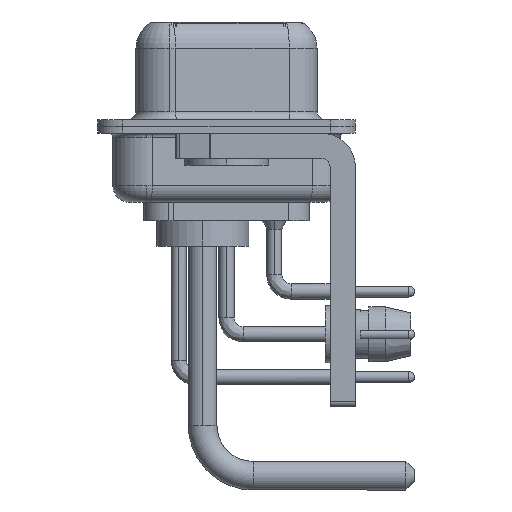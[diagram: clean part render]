
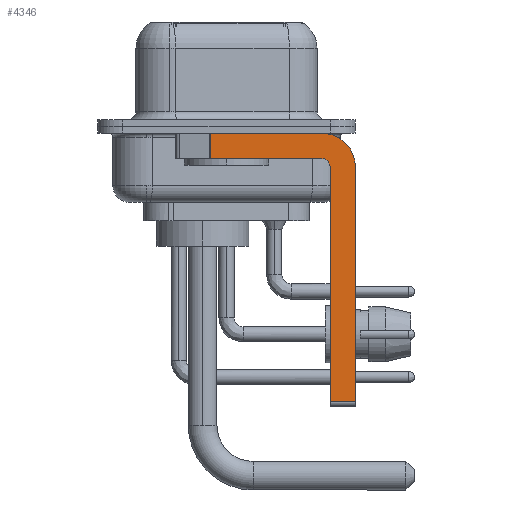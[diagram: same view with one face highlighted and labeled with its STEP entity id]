
A CAD part, left-side view. The second image highlights one B-rep face of the part: STEP entity #4346.
In plain terms, the highlighted planar face has unit normal (-1, 0, 0).
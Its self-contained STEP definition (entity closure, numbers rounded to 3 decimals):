
#274 = EDGE_CURVE ( 'NONE', #16400, #15756, #26025, .T. ) ;
#583 = EDGE_CURVE ( 'NONE', #9301, #2854, #10299, .T. ) ;
#618 = EDGE_CURVE ( 'NONE', #28254, #19054, #13536, .T. ) ;
#1569 = EDGE_CURVE ( 'NONE', #19054, #15756, #11273, .T. ) ;
#2556 = PLANE ( 'NONE',  #16805 ) ;
#2561 = VERTEX_POINT ( 'NONE', #9936 ) ;
#2715 = DIRECTION ( 'NONE',  ( 0., 0., 1. ) ) ;
#2854 = VERTEX_POINT ( 'NONE', #19537 ) ;
#3910 = DIRECTION ( 'NONE',  ( 0., 1., 0. ) ) ;
#4150 = EDGE_CURVE ( 'NONE', #2561, #2854, #21300, .T. ) ;
#4299 = VECTOR ( 'NONE', #22179, 1000. ) ;
#4346 = ADVANCED_FACE ( 'NONE', ( #14711 ), #2556, .F. ) ;
#4815 = ORIENTED_EDGE ( 'NONE', *, *, #618, .F. ) ;
#4873 = DIRECTION ( 'NONE',  ( 1., 0., 0. ) ) ;
#5376 = AXIS2_PLACEMENT_3D ( 'NONE', #22661, #20247, #10449 ) ;
#5695 = VECTOR ( 'NONE', #3910, 1000. ) ;
#6154 = CARTESIAN_POINT ( 'NONE',  ( -2.9, 0.978, -1.9 ) ) ;
#6637 = VECTOR ( 'NONE', #8551, 1000. ) ;
#7139 = VECTOR ( 'NONE', #14784, 1000. ) ;
#8011 = ORIENTED_EDGE ( 'NONE', *, *, #20557, .F. ) ;
#8551 = DIRECTION ( 'NONE',  ( 0., 0., -1. ) ) ;
#8844 = CIRCLE ( 'NONE', #9340, 2. ) ;
#9301 = VERTEX_POINT ( 'NONE', #30287 ) ;
#9340 = AXIS2_PLACEMENT_3D ( 'NONE', #26995, #4873, #14967 ) ;
#9581 = DIRECTION ( 'NONE',  ( 1., 0., 0. ) ) ;
#9936 = CARTESIAN_POINT ( 'NONE',  ( -2.9, -7.65, -2.4 ) ) ;
#9982 = CARTESIAN_POINT ( 'NONE',  ( -2.9, -5.65, -16.35 ) ) ;
#9999 = EDGE_CURVE ( 'NONE', #9301, #28254, #22275, .T. ) ;
#10299 = LINE ( 'NONE', #9982, #4299 ) ;
#10449 = DIRECTION ( 'NONE',  ( 0., 0., 1. ) ) ;
#10616 = VECTOR ( 'NONE', #16011, 1000. ) ;
#10702 = VERTEX_POINT ( 'NONE', #15596 ) ;
#10873 = CARTESIAN_POINT ( 'NONE',  ( -2.9, -7.65, -2.4 ) ) ;
#10955 = CARTESIAN_POINT ( 'NONE',  ( -2.9, -5.65, -1.9 ) ) ;
#11273 = LINE ( 'NONE', #10955, #5695 ) ;
#12089 = CARTESIAN_POINT ( 'NONE',  ( -2.9, -6.15, -2.4 ) ) ;
#12495 = ORIENTED_EDGE ( 'NONE', *, *, #1569, .F. ) ;
#13536 = CIRCLE ( 'NONE', #5376, 0.5 ) ;
#14338 = ORIENTED_EDGE ( 'NONE', *, *, #4150, .F. ) ;
#14711 = FACE_OUTER_BOUND ( 'NONE', #17903, .T. ) ;
#14784 = DIRECTION ( 'NONE',  ( 0., -1., 0. ) ) ;
#14967 = DIRECTION ( 'NONE',  ( 0., 0., -1. ) ) ;
#15596 = CARTESIAN_POINT ( 'NONE',  ( -2.9, -5.65, -0.4 ) ) ;
#15642 = ORIENTED_EDGE ( 'NONE', *, *, #583, .T. ) ;
#15756 = VERTEX_POINT ( 'NONE', #29394 ) ;
#16011 = DIRECTION ( 'NONE',  ( 0., 0., -1. ) ) ;
#16400 = VERTEX_POINT ( 'NONE', #18113 ) ;
#16805 = AXIS2_PLACEMENT_3D ( 'NONE', #31576, #9581, #19217 ) ;
#17903 = EDGE_LOOP ( 'NONE', ( #8011, #23789, #12495, #4815, #29987, #15642, #14338, #29711 ) ) ;
#18113 = CARTESIAN_POINT ( 'NONE',  ( -2.9, 0.978, -0.4 ) ) ;
#19054 = VERTEX_POINT ( 'NONE', #31001 ) ;
#19217 = DIRECTION ( 'NONE',  ( 0., 0., -1. ) ) ;
#19537 = CARTESIAN_POINT ( 'NONE',  ( -2.9, -7.65, -16.35 ) ) ;
#20247 = DIRECTION ( 'NONE',  ( -1., 0., 0. ) ) ;
#20557 = EDGE_CURVE ( 'NONE', #16400, #10702, #24577, .T. ) ;
#21300 = LINE ( 'NONE', #10873, #10616 ) ;
#22179 = DIRECTION ( 'NONE',  ( 0., -1., 0. ) ) ;
#22275 = LINE ( 'NONE', #24514, #26876 ) ;
#22661 = CARTESIAN_POINT ( 'NONE',  ( -2.9, -5.65, -2.4 ) ) ;
#23789 = ORIENTED_EDGE ( 'NONE', *, *, #274, .T. ) ;
#23838 = EDGE_CURVE ( 'NONE', #10702, #2561, #8844, .T. ) ;
#24514 = CARTESIAN_POINT ( 'NONE',  ( -2.9, -6.15, -16.6 ) ) ;
#24577 = LINE ( 'NONE', #26652, #7139 ) ;
#26025 = LINE ( 'NONE', #6154, #6637 ) ;
#26652 = CARTESIAN_POINT ( 'NONE',  ( -2.9, 3., -0.4 ) ) ;
#26876 = VECTOR ( 'NONE', #2715, 1000. ) ;
#26995 = CARTESIAN_POINT ( 'NONE',  ( -2.9, -5.65, -2.4 ) ) ;
#28254 = VERTEX_POINT ( 'NONE', #12089 ) ;
#29394 = CARTESIAN_POINT ( 'NONE',  ( -2.9, 0.978, -1.9 ) ) ;
#29711 = ORIENTED_EDGE ( 'NONE', *, *, #23838, .F. ) ;
#29987 = ORIENTED_EDGE ( 'NONE', *, *, #9999, .F. ) ;
#30287 = CARTESIAN_POINT ( 'NONE',  ( -2.9, -6.15, -16.35 ) ) ;
#31001 = CARTESIAN_POINT ( 'NONE',  ( -2.9, -5.65, -1.9 ) ) ;
#31576 = CARTESIAN_POINT ( 'NONE',  ( -2.9, -5.65, -2.4 ) ) ;
